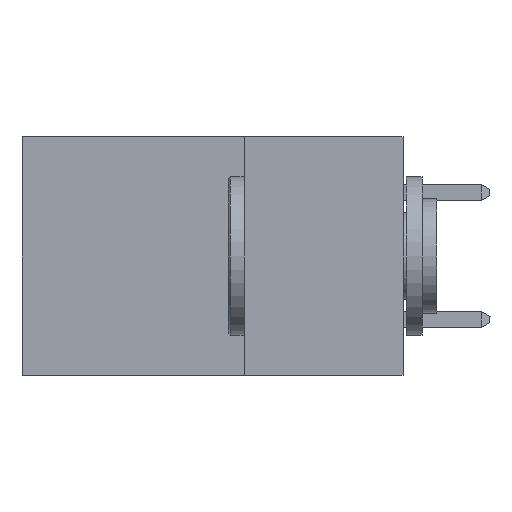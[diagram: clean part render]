
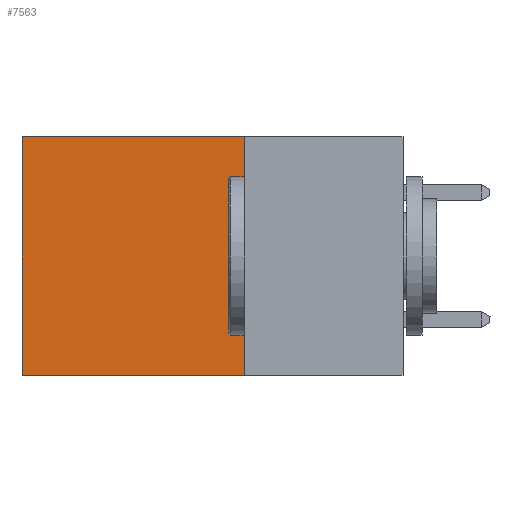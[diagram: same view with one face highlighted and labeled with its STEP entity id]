
A CAD part, left-side view. The second image highlights one B-rep face of the part: STEP entity #7563.
In plain terms, the highlighted planar face has unit normal (-1, 0, 0).
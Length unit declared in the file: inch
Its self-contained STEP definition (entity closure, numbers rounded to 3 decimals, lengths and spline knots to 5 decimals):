
#721 = CARTESIAN_POINT ( 'NONE',  ( 0.2875, 0.6, -0.375 ) ) ;
#1609 = DIRECTION ( 'NONE',  ( 0., 1., 0. ) ) ;
#2416 = LINE ( 'NONE', #18814, #17416 ) ;
#3059 = DIRECTION ( 'NONE',  ( 1., 0., 0. ) ) ;
#3080 = LINE ( 'NONE', #15797, #11277 ) ;
#3122 = VERTEX_POINT ( 'NONE', #15541 ) ;
#3314 = VECTOR ( 'NONE', #18503, 39.37008 ) ;
#3583 = EDGE_CURVE ( 'NONE', #6573, #16667, #15801, .T. ) ;
#4587 = PLANE ( 'NONE',  #11206 ) ;
#4736 = CARTESIAN_POINT ( 'NONE',  ( 0.2875, 0.25, -0.375 ) ) ;
#5431 = ORIENTED_EDGE ( 'NONE', *, *, #11820, .F. ) ;
#6486 = VERTEX_POINT ( 'NONE', #21689 ) ;
#6573 = VERTEX_POINT ( 'NONE', #14254 ) ;
#7563 = ADVANCED_FACE ( 'NONE', ( #8544 ), #4587, .F. ) ;
#8397 = EDGE_LOOP ( 'NONE', ( #18451, #5431, #21225, #18733 ) ) ;
#8507 = CARTESIAN_POINT ( 'NONE',  ( 0.2875, 0.6, -0.375 ) ) ;
#8533 = EDGE_CURVE ( 'NONE', #6486, #3122, #11521, .T. ) ;
#8544 = FACE_OUTER_BOUND ( 'NONE', #8397, .T. ) ;
#11206 = AXIS2_PLACEMENT_3D ( 'NONE', #18710, #3059, #16788 ) ;
#11277 = VECTOR ( 'NONE', #1609, 39.37008 ) ;
#11521 = LINE ( 'NONE', #4736, #3314 ) ;
#11820 = EDGE_CURVE ( 'NONE', #3122, #16667, #3080, .T. ) ;
#13360 = VECTOR ( 'NONE', #14935, 39.37008 ) ;
#14254 = CARTESIAN_POINT ( 'NONE',  ( 0.2875, 0.6, 0. ) ) ;
#14935 = DIRECTION ( 'NONE',  ( 0., 0., -1. ) ) ;
#15171 = EDGE_CURVE ( 'NONE', #6486, #6573, #2416, .T. ) ;
#15541 = CARTESIAN_POINT ( 'NONE',  ( 0.2875, 0.25, -0.375 ) ) ;
#15797 = CARTESIAN_POINT ( 'NONE',  ( 0.2875, 0.25, -0.375 ) ) ;
#15801 = LINE ( 'NONE', #721, #13360 ) ;
#16667 = VERTEX_POINT ( 'NONE', #8507 ) ;
#16746 = DIRECTION ( 'NONE',  ( 0., 1., 0. ) ) ;
#16788 = DIRECTION ( 'NONE',  ( 0., 0., -1. ) ) ;
#17416 = VECTOR ( 'NONE', #16746, 39.37008 ) ;
#18451 = ORIENTED_EDGE ( 'NONE', *, *, #3583, .T. ) ;
#18503 = DIRECTION ( 'NONE',  ( 0., 0., -1. ) ) ;
#18710 = CARTESIAN_POINT ( 'NONE',  ( 0.2875, 0.25, -0.375 ) ) ;
#18733 = ORIENTED_EDGE ( 'NONE', *, *, #15171, .T. ) ;
#18814 = CARTESIAN_POINT ( 'NONE',  ( 0.2875, 0.25, 0. ) ) ;
#21225 = ORIENTED_EDGE ( 'NONE', *, *, #8533, .F. ) ;
#21689 = CARTESIAN_POINT ( 'NONE',  ( 0.2875, 0.25, 0. ) ) ;
